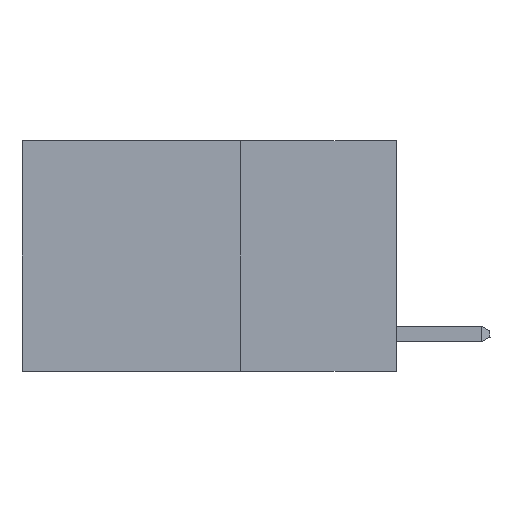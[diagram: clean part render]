
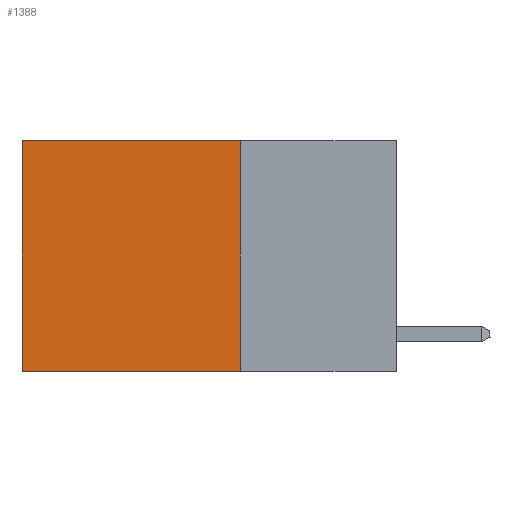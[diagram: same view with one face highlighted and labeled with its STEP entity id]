
A CAD part, left-side view. The second image highlights one B-rep face of the part: STEP entity #1388.
In plain terms, the highlighted planar face has unit normal (-1, 0, 0).
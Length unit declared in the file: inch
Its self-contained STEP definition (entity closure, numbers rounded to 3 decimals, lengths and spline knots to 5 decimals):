
#856 = VERTEX_POINT ( 'NONE', #10459 ) ;
#1388 = ADVANCED_FACE ( 'NONE', ( #13924 ), #3991, .F. ) ;
#1728 = CARTESIAN_POINT ( 'NONE',  ( 0.2625, 0.25, 0. ) ) ;
#1780 = VECTOR ( 'NONE', #17748, 39.37008 ) ;
#1882 = CARTESIAN_POINT ( 'NONE',  ( 0.2625, 0.25, 0. ) ) ;
#2366 = ORIENTED_EDGE ( 'NONE', *, *, #11138, .F. ) ;
#2808 = ORIENTED_EDGE ( 'NONE', *, *, #7684, .T. ) ;
#2823 = EDGE_CURVE ( 'NONE', #856, #20788, #18157, .T. ) ;
#3185 = CARTESIAN_POINT ( 'NONE',  ( 0.2625, 0.25, 0. ) ) ;
#3806 = DIRECTION ( 'NONE',  ( 0., 0., -1. ) ) ;
#3901 = DIRECTION ( 'NONE',  ( 1., 0., 0. ) ) ;
#3920 = CARTESIAN_POINT ( 'NONE',  ( 0.2625, 0.25, 0. ) ) ;
#3991 = PLANE ( 'NONE',  #7538 ) ;
#5026 = VECTOR ( 'NONE', #14994, 39.37008 ) ;
#6779 = DIRECTION ( 'NONE',  ( 0., 1., 0. ) ) ;
#7538 = AXIS2_PLACEMENT_3D ( 'NONE', #3920, #3901, #3806 ) ;
#7684 = EDGE_CURVE ( 'NONE', #16605, #856, #20295, .T. ) ;
#7941 = CARTESIAN_POINT ( 'NONE',  ( 0.2625, 0.25, -0.37 ) ) ;
#10459 = CARTESIAN_POINT ( 'NONE',  ( 0.2625, 0.6, 0. ) ) ;
#11138 = EDGE_CURVE ( 'NONE', #16605, #19673, #19898, .T. ) ;
#11299 = ORIENTED_EDGE ( 'NONE', *, *, #2823, .T. ) ;
#11696 = CARTESIAN_POINT ( 'NONE',  ( 0.2625, 0.6, 0. ) ) ;
#12170 = VECTOR ( 'NONE', #6779, 39.37008 ) ;
#13924 = FACE_OUTER_BOUND ( 'NONE', #16008, .T. ) ;
#14485 = ORIENTED_EDGE ( 'NONE', *, *, #19630, .F. ) ;
#14994 = DIRECTION ( 'NONE',  ( 0., 0., -1. ) ) ;
#15599 = VECTOR ( 'NONE', #16388, 39.37008 ) ;
#16008 = EDGE_LOOP ( 'NONE', ( #11299, #14485, #2366, #2808 ) ) ;
#16125 = CARTESIAN_POINT ( 'NONE',  ( 0.2625, 0.25, -0.37 ) ) ;
#16388 = DIRECTION ( 'NONE',  ( 0., 0., -1. ) ) ;
#16605 = VERTEX_POINT ( 'NONE', #1882 ) ;
#17252 = CARTESIAN_POINT ( 'NONE',  ( 0.2625, 0.6, -0.37 ) ) ;
#17748 = DIRECTION ( 'NONE',  ( 0., 1., 0. ) ) ;
#18157 = LINE ( 'NONE', #11696, #5026 ) ;
#19363 = LINE ( 'NONE', #16125, #1780 ) ;
#19630 = EDGE_CURVE ( 'NONE', #19673, #20788, #19363, .T. ) ;
#19673 = VERTEX_POINT ( 'NONE', #7941 ) ;
#19898 = LINE ( 'NONE', #3185, #15599 ) ;
#20295 = LINE ( 'NONE', #1728, #12170 ) ;
#20788 = VERTEX_POINT ( 'NONE', #17252 ) ;
